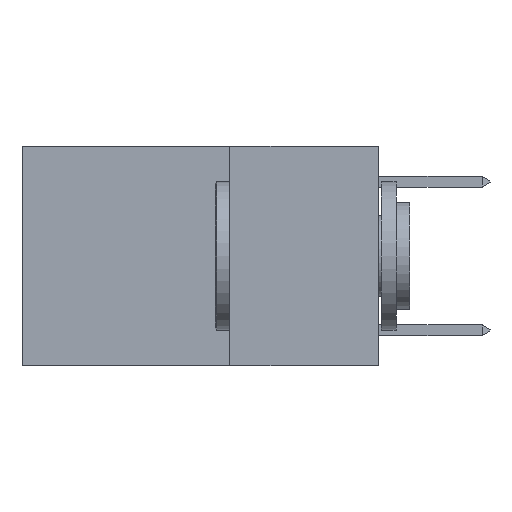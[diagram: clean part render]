
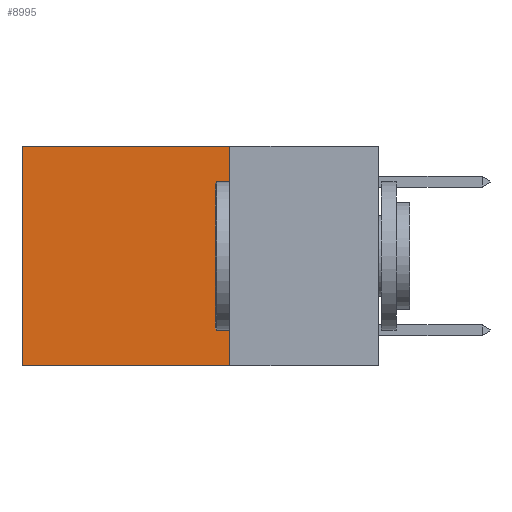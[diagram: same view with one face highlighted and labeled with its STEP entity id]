
A CAD part, left-side view. The second image highlights one B-rep face of the part: STEP entity #8995.
In plain terms, the highlighted planar face has unit normal (-1, 0, 0).
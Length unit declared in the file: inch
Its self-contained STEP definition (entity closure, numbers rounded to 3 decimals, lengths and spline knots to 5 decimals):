
#590 = DIRECTION ( 'NONE',  ( 0., 0., -1. ) ) ;
#1007 = CARTESIAN_POINT ( 'NONE',  ( 0.2625, 0.25, 0. ) ) ;
#1029 = EDGE_CURVE ( 'NONE', #5645, #9169, #5535, .T. ) ;
#1841 = VECTOR ( 'NONE', #590, 39.37008 ) ;
#2087 = LINE ( 'NONE', #3881, #6006 ) ;
#2225 = VERTEX_POINT ( 'NONE', #10471 ) ;
#2478 = LINE ( 'NONE', #5272, #7455 ) ;
#2875 = PLANE ( 'NONE',  #8300 ) ;
#2894 = CARTESIAN_POINT ( 'NONE',  ( 0.2625, 0.25, 0. ) ) ;
#3421 = DIRECTION ( 'NONE',  ( 0., 0., -1. ) ) ;
#3544 = VECTOR ( 'NONE', #7960, 39.37008 ) ;
#3881 = CARTESIAN_POINT ( 'NONE',  ( 0.2625, 0.25, -0.37 ) ) ;
#4313 = ORIENTED_EDGE ( 'NONE', *, *, #1029, .T. ) ;
#4616 = FACE_OUTER_BOUND ( 'NONE', #9681, .T. ) ;
#4637 = EDGE_CURVE ( 'NONE', #5645, #10147, #2478, .T. ) ;
#5156 = EDGE_CURVE ( 'NONE', #10147, #2225, #2087, .T. ) ;
#5272 = CARTESIAN_POINT ( 'NONE',  ( 0.2625, 0.25, 0. ) ) ;
#5535 = LINE ( 'NONE', #9130, #3544 ) ;
#5645 = VERTEX_POINT ( 'NONE', #2894 ) ;
#6006 = VECTOR ( 'NONE', #7412, 39.37008 ) ;
#6240 = CARTESIAN_POINT ( 'NONE',  ( 0.2625, 0.25, -0.37 ) ) ;
#6965 = CARTESIAN_POINT ( 'NONE',  ( 0.2625, 0.6, 0. ) ) ;
#7387 = DIRECTION ( 'NONE',  ( 1., 0., 0. ) ) ;
#7412 = DIRECTION ( 'NONE',  ( 0., 1., 0. ) ) ;
#7455 = VECTOR ( 'NONE', #3421, 39.37008 ) ;
#7960 = DIRECTION ( 'NONE',  ( 0., 1., 0. ) ) ;
#8268 = DIRECTION ( 'NONE',  ( 0., 0., -1. ) ) ;
#8300 = AXIS2_PLACEMENT_3D ( 'NONE', #1007, #7387, #8268 ) ;
#8558 = LINE ( 'NONE', #9613, #1841 ) ;
#8661 = ORIENTED_EDGE ( 'NONE', *, *, #9953, .T. ) ;
#8995 = ADVANCED_FACE ( 'NONE', ( #4616 ), #2875, .F. ) ;
#9076 = ORIENTED_EDGE ( 'NONE', *, *, #4637, .F. ) ;
#9130 = CARTESIAN_POINT ( 'NONE',  ( 0.2625, 0.25, 0. ) ) ;
#9169 = VERTEX_POINT ( 'NONE', #6965 ) ;
#9613 = CARTESIAN_POINT ( 'NONE',  ( 0.2625, 0.6, 0. ) ) ;
#9681 = EDGE_LOOP ( 'NONE', ( #8661, #10473, #9076, #4313 ) ) ;
#9953 = EDGE_CURVE ( 'NONE', #9169, #2225, #8558, .T. ) ;
#10147 = VERTEX_POINT ( 'NONE', #6240 ) ;
#10471 = CARTESIAN_POINT ( 'NONE',  ( 0.2625, 0.6, -0.37 ) ) ;
#10473 = ORIENTED_EDGE ( 'NONE', *, *, #5156, .F. ) ;
